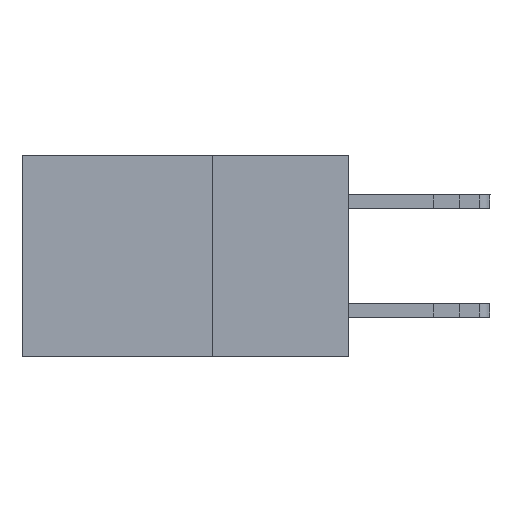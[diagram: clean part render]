
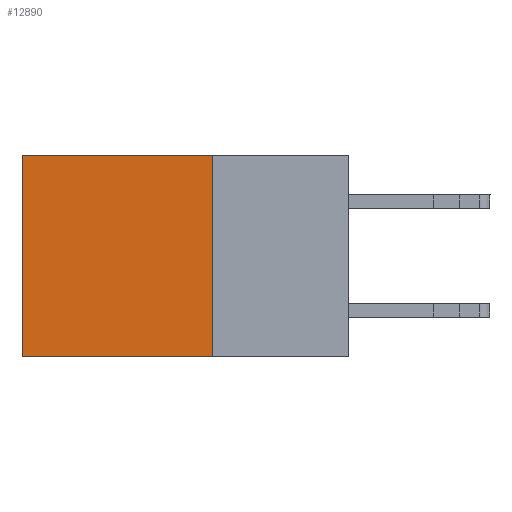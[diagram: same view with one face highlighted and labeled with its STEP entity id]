
A CAD part, left-side view. The second image highlights one B-rep face of the part: STEP entity #12890.
In plain terms, the highlighted planar face has unit normal (-1, 0, 0).
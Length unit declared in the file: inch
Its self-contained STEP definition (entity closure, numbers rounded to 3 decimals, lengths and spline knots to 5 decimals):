
#689 = CARTESIAN_POINT ( 'NONE',  ( 0.298, 0.6, 0. ) ) ;
#1753 = EDGE_CURVE ( 'NONE', #7835, #13511, #2942, .T. ) ;
#1880 = LINE ( 'NONE', #689, #9635 ) ;
#1938 = FACE_OUTER_BOUND ( 'NONE', #14981, .T. ) ;
#2534 = VECTOR ( 'NONE', #7768, 39.37008 ) ;
#2848 = CARTESIAN_POINT ( 'NONE',  ( 0.298, 0.25, 0. ) ) ;
#2942 = LINE ( 'NONE', #12452, #2534 ) ;
#2962 = CARTESIAN_POINT ( 'NONE',  ( 0.298, 0.25, 0. ) ) ;
#3088 = VECTOR ( 'NONE', #12014, 39.37008 ) ;
#4473 = CARTESIAN_POINT ( 'NONE',  ( 0.298, 0.6, 0. ) ) ;
#4700 = EDGE_CURVE ( 'NONE', #15524, #13511, #1880, .T. ) ;
#5403 = ORIENTED_EDGE ( 'NONE', *, *, #15434, .T. ) ;
#5508 = DIRECTION ( 'NONE',  ( 0., 0., -1. ) ) ;
#6771 = DIRECTION ( 'NONE',  ( 1., 0., 0. ) ) ;
#7306 = CARTESIAN_POINT ( 'NONE',  ( 0.298, 0.25, -0.37 ) ) ;
#7639 = PLANE ( 'NONE',  #15186 ) ;
#7669 = VECTOR ( 'NONE', #9214, 39.37008 ) ;
#7768 = DIRECTION ( 'NONE',  ( 0., 1., 0. ) ) ;
#7835 = VERTEX_POINT ( 'NONE', #7306 ) ;
#7958 = DIRECTION ( 'NONE',  ( 0., 0., -1. ) ) ;
#8004 = LINE ( 'NONE', #15556, #3088 ) ;
#8056 = ORIENTED_EDGE ( 'NONE', *, *, #4700, .T. ) ;
#9214 = DIRECTION ( 'NONE',  ( 0., 1., 0. ) ) ;
#9635 = VECTOR ( 'NONE', #5508, 39.37008 ) ;
#9685 = ORIENTED_EDGE ( 'NONE', *, *, #13706, .F. ) ;
#11100 = VERTEX_POINT ( 'NONE', #2848 ) ;
#12014 = DIRECTION ( 'NONE',  ( 0., 0., -1. ) ) ;
#12452 = CARTESIAN_POINT ( 'NONE',  ( 0.298, 0.25, -0.37 ) ) ;
#12458 = ORIENTED_EDGE ( 'NONE', *, *, #1753, .F. ) ;
#12890 = ADVANCED_FACE ( 'NONE', ( #1938 ), #7639, .F. ) ;
#13511 = VERTEX_POINT ( 'NONE', #13678 ) ;
#13678 = CARTESIAN_POINT ( 'NONE',  ( 0.298, 0.6, -0.37 ) ) ;
#13706 = EDGE_CURVE ( 'NONE', #11100, #7835, #8004, .T. ) ;
#13742 = LINE ( 'NONE', #15308, #7669 ) ;
#14981 = EDGE_LOOP ( 'NONE', ( #8056, #12458, #9685, #5403 ) ) ;
#15186 = AXIS2_PLACEMENT_3D ( 'NONE', #2962, #6771, #7958 ) ;
#15308 = CARTESIAN_POINT ( 'NONE',  ( 0.298, 0.25, 0. ) ) ;
#15434 = EDGE_CURVE ( 'NONE', #11100, #15524, #13742, .T. ) ;
#15524 = VERTEX_POINT ( 'NONE', #4473 ) ;
#15556 = CARTESIAN_POINT ( 'NONE',  ( 0.298, 0.25, 0. ) ) ;
